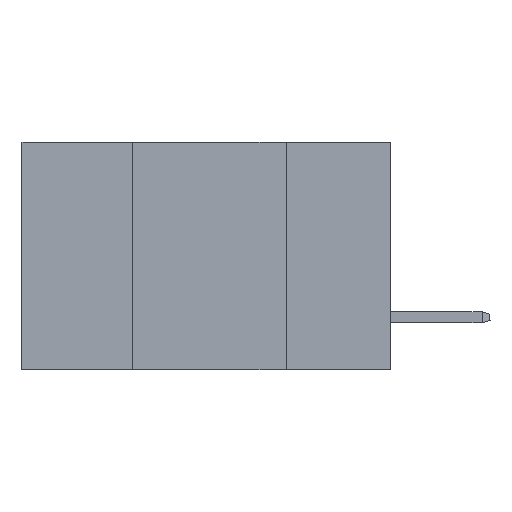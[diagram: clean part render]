
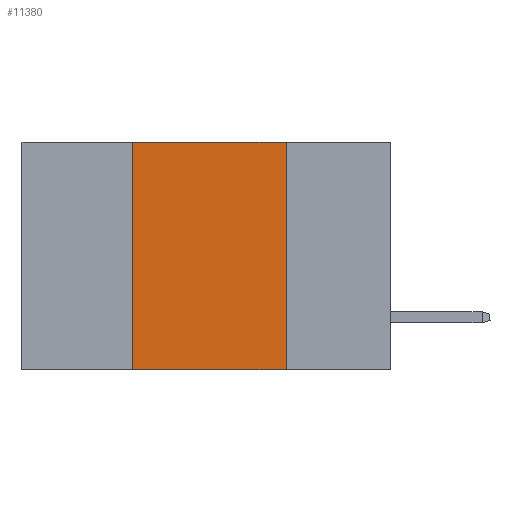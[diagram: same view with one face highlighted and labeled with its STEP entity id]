
A CAD part, left-side view. The second image highlights one B-rep face of the part: STEP entity #11380.
In plain terms, the highlighted planar face has unit normal (-1, 0, 0).
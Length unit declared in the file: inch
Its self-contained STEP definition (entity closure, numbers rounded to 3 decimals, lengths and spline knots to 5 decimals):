
#1316 = PLANE ( 'NONE',  #20530 ) ;
#1460 = VERTEX_POINT ( 'NONE', #3905 ) ;
#1487 = FACE_OUTER_BOUND ( 'NONE', #5281, .T. ) ;
#2434 = VECTOR ( 'NONE', #22362, 39.37008 ) ;
#3029 = VECTOR ( 'NONE', #18709, 39.37008 ) ;
#3905 = CARTESIAN_POINT ( 'NONE',  ( 0., 0.17, 0. ) ) ;
#3947 = CARTESIAN_POINT ( 'NONE',  ( 0., 0.6, -0.37 ) ) ;
#5281 = EDGE_LOOP ( 'NONE', ( #6242, #13826, #14105, #12974 ) ) ;
#5326 = EDGE_CURVE ( 'NONE', #14248, #16849, #11308, .T. ) ;
#5827 = DIRECTION ( 'NONE',  ( 0., 0., 1. ) ) ;
#6242 = ORIENTED_EDGE ( 'NONE', *, *, #20917, .F. ) ;
#6272 = VECTOR ( 'NONE', #5827, 39.37008 ) ;
#6538 = LINE ( 'NONE', #17281, #3029 ) ;
#6902 = EDGE_CURVE ( 'NONE', #14248, #13491, #15023, .T. ) ;
#9887 = DIRECTION ( 'NONE',  ( 0., 0., -1. ) ) ;
#10160 = CARTESIAN_POINT ( 'NONE',  ( 0., 0.6, 0. ) ) ;
#11308 = LINE ( 'NONE', #3947, #16757 ) ;
#11380 = ADVANCED_FACE ( 'NONE', ( #1487 ), #1316, .F. ) ;
#12088 = CARTESIAN_POINT ( 'NONE',  ( 0., 0.42, 0. ) ) ;
#12223 = LINE ( 'NONE', #10160, #2434 ) ;
#12974 = ORIENTED_EDGE ( 'NONE', *, *, #5326, .T. ) ;
#12978 = DIRECTION ( 'NONE',  ( 0., -1., 0. ) ) ;
#13491 = VERTEX_POINT ( 'NONE', #12088 ) ;
#13826 = ORIENTED_EDGE ( 'NONE', *, *, #21656, .F. ) ;
#14105 = ORIENTED_EDGE ( 'NONE', *, *, #6902, .F. ) ;
#14248 = VERTEX_POINT ( 'NONE', #16960 ) ;
#15023 = LINE ( 'NONE', #21291, #6272 ) ;
#16757 = VECTOR ( 'NONE', #12978, 39.37008 ) ;
#16849 = VERTEX_POINT ( 'NONE', #20893 ) ;
#16960 = CARTESIAN_POINT ( 'NONE',  ( 0., 0.42, -0.37 ) ) ;
#17130 = CARTESIAN_POINT ( 'NONE',  ( 0., 0.6, 0. ) ) ;
#17281 = CARTESIAN_POINT ( 'NONE',  ( 0., 0.17, 0. ) ) ;
#18709 = DIRECTION ( 'NONE',  ( 0., 0., -1. ) ) ;
#20333 = DIRECTION ( 'NONE',  ( 1., 0., 0. ) ) ;
#20530 = AXIS2_PLACEMENT_3D ( 'NONE', #17130, #20333, #9887 ) ;
#20893 = CARTESIAN_POINT ( 'NONE',  ( 0., 0.17, -0.37 ) ) ;
#20917 = EDGE_CURVE ( 'NONE', #1460, #16849, #6538, .T. ) ;
#21291 = CARTESIAN_POINT ( 'NONE',  ( 0., 0.42, 0. ) ) ;
#21656 = EDGE_CURVE ( 'NONE', #13491, #1460, #12223, .T. ) ;
#22362 = DIRECTION ( 'NONE',  ( 0., -1., 0. ) ) ;
